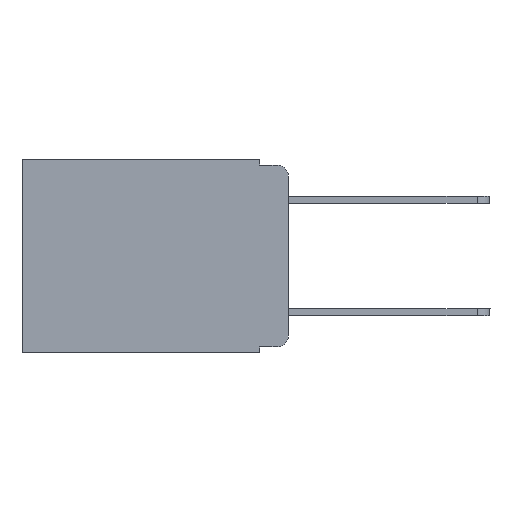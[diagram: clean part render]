
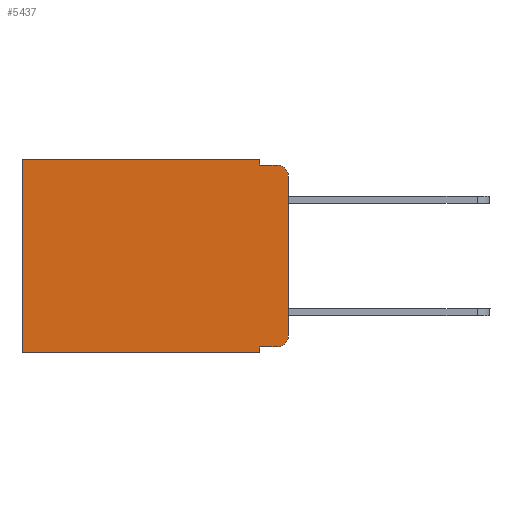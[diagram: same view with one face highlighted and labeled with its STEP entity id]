
A CAD part, left-side view. The second image highlights one B-rep face of the part: STEP entity #5437.
In plain terms, the highlighted planar face has unit normal (-1, 0, 0).
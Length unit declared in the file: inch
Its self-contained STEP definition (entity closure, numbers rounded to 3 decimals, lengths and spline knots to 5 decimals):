
#81 = CIRCLE ( 'NONE', #7023, 0.02 ) ;
#609 = CARTESIAN_POINT ( 'NONE',  ( 0.298, 0., 0. ) ) ;
#875 = DIRECTION ( 'NONE',  ( -1., 0., 0. ) ) ;
#1164 = CARTESIAN_POINT ( 'NONE',  ( 0.298, 0., -0.313 ) ) ;
#1168 = EDGE_CURVE ( 'NONE', #8447, #5330, #4575, .T. ) ;
#1193 = ORIENTED_EDGE ( 'NONE', *, *, #2212, .T. ) ;
#1303 = DIRECTION ( 'NONE',  ( 0., 0., -1. ) ) ;
#1334 = DIRECTION ( 'NONE',  ( 0., 0., -1. ) ) ;
#1465 = LINE ( 'NONE', #5973, #4392 ) ;
#1479 = ORIENTED_EDGE ( 'NONE', *, *, #4085, .F. ) ;
#1498 = DIRECTION ( 'NONE',  ( 0., 0., -1. ) ) ;
#1817 = CARTESIAN_POINT ( 'NONE',  ( 0.298, 0.02, -0.313 ) ) ;
#1825 = EDGE_CURVE ( 'NONE', #5788, #2745, #9775, .T. ) ;
#2212 = EDGE_CURVE ( 'NONE', #3361, #5788, #9214, .T. ) ;
#2239 = ORIENTED_EDGE ( 'NONE', *, *, #1168, .F. ) ;
#2582 = CARTESIAN_POINT ( 'NONE',  ( 0.298, 0.051, -0.333 ) ) ;
#2745 = VERTEX_POINT ( 'NONE', #1164 ) ;
#2805 = LINE ( 'NONE', #609, #9180 ) ;
#2934 = CARTESIAN_POINT ( 'NONE',  ( 0.298, 0.02, -0.03 ) ) ;
#2953 = ORIENTED_EDGE ( 'NONE', *, *, #7912, .T. ) ;
#3233 = LINE ( 'NONE', #3940, #7181 ) ;
#3247 = EDGE_CURVE ( 'NONE', #8263, #9102, #1465, .T. ) ;
#3316 = AXIS2_PLACEMENT_3D ( 'NONE', #1817, #875, #8660 ) ;
#3361 = VERTEX_POINT ( 'NONE', #7774 ) ;
#3495 = DIRECTION ( 'NONE',  ( 0., -1., 0. ) ) ;
#3510 = ORIENTED_EDGE ( 'NONE', *, *, #8692, .F. ) ;
#3664 = VECTOR ( 'NONE', #3495, 39.37008 ) ;
#3793 = CARTESIAN_POINT ( 'NONE',  ( 0.298, 0.051, 0. ) ) ;
#3894 = LINE ( 'NONE', #3793, #7032 ) ;
#3940 = CARTESIAN_POINT ( 'NONE',  ( 0.298, 0., 0. ) ) ;
#4006 = PLANE ( 'NONE',  #4125 ) ;
#4085 = EDGE_CURVE ( 'NONE', #3361, #9686, #7409, .T. ) ;
#4125 = AXIS2_PLACEMENT_3D ( 'NONE', #9094, #4839, #10782 ) ;
#4205 = ORIENTED_EDGE ( 'NONE', *, *, #1825, .T. ) ;
#4349 = CARTESIAN_POINT ( 'NONE',  ( 0.298, 0.473, 0. ) ) ;
#4392 = VECTOR ( 'NONE', #6828, 39.37008 ) ;
#4540 = DIRECTION ( 'NONE',  ( 0., 0., -1. ) ) ;
#4575 = LINE ( 'NONE', #6539, #10565 ) ;
#4653 = DIRECTION ( 'NONE',  ( -1., 0., 0. ) ) ;
#4718 = EDGE_LOOP ( 'NONE', ( #10813, #7399, #2239, #9500, #2953, #8343, #3510, #1479, #1193, #4205 ) ) ;
#4820 = EDGE_CURVE ( 'NONE', #7553, #2745, #2805, .T. ) ;
#4839 = DIRECTION ( 'NONE',  ( 1., 0., 0. ) ) ;
#4878 = DIRECTION ( 'NONE',  ( 0., -1., 0. ) ) ;
#5330 = VERTEX_POINT ( 'NONE', #10750 ) ;
#5437 = ADVANCED_FACE ( 'NONE', ( #6468 ), #4006, .F. ) ;
#5440 = CARTESIAN_POINT ( 'NONE',  ( 0.298, 0.051, -0.343 ) ) ;
#5788 = VERTEX_POINT ( 'NONE', #8857 ) ;
#5789 = EDGE_CURVE ( 'NONE', #7553, #5330, #81, .T. ) ;
#5932 = DIRECTION ( 'NONE',  ( 0., 1., 0. ) ) ;
#5973 = CARTESIAN_POINT ( 'NONE',  ( 0.298, 0.473, 0. ) ) ;
#6303 = CARTESIAN_POINT ( 'NONE',  ( 0.298, 0.051, 0. ) ) ;
#6416 = CARTESIAN_POINT ( 'NONE',  ( 0.298, 0.473, -0.343 ) ) ;
#6468 = FACE_OUTER_BOUND ( 'NONE', #4718, .T. ) ;
#6539 = CARTESIAN_POINT ( 'NONE',  ( 0.298, 0.051, -0.01 ) ) ;
#6828 = DIRECTION ( 'NONE',  ( 0., 0., -1. ) ) ;
#7023 = AXIS2_PLACEMENT_3D ( 'NONE', #2934, #4653, #1303 ) ;
#7032 = VECTOR ( 'NONE', #4540, 39.37008 ) ;
#7159 = VECTOR ( 'NONE', #1334, 39.37008 ) ;
#7181 = VECTOR ( 'NONE', #7205, 39.37008 ) ;
#7205 = DIRECTION ( 'NONE',  ( 0., 1., 0. ) ) ;
#7399 = ORIENTED_EDGE ( 'NONE', *, *, #5789, .T. ) ;
#7409 = LINE ( 'NONE', #6303, #7159 ) ;
#7553 = VERTEX_POINT ( 'NONE', #9924 ) ;
#7774 = CARTESIAN_POINT ( 'NONE',  ( 0.298, 0.051, -0.333 ) ) ;
#7912 = EDGE_CURVE ( 'NONE', #10568, #8263, #3233, .T. ) ;
#8120 = VECTOR ( 'NONE', #5932, 39.37008 ) ;
#8263 = VERTEX_POINT ( 'NONE', #4349 ) ;
#8343 = ORIENTED_EDGE ( 'NONE', *, *, #3247, .T. ) ;
#8447 = VERTEX_POINT ( 'NONE', #9722 ) ;
#8660 = DIRECTION ( 'NONE',  ( 0., 0., -1. ) ) ;
#8692 = EDGE_CURVE ( 'NONE', #9686, #9102, #10400, .T. ) ;
#8711 = CARTESIAN_POINT ( 'NONE',  ( 0.298, 0.051, 0. ) ) ;
#8857 = CARTESIAN_POINT ( 'NONE',  ( 0.298, 0.02, -0.333 ) ) ;
#8982 = EDGE_CURVE ( 'NONE', #10568, #8447, #3894, .T. ) ;
#9094 = CARTESIAN_POINT ( 'NONE',  ( 0.298, 0., 0. ) ) ;
#9102 = VERTEX_POINT ( 'NONE', #6416 ) ;
#9180 = VECTOR ( 'NONE', #1498, 39.37008 ) ;
#9214 = LINE ( 'NONE', #2582, #3664 ) ;
#9500 = ORIENTED_EDGE ( 'NONE', *, *, #8982, .F. ) ;
#9686 = VERTEX_POINT ( 'NONE', #5440 ) ;
#9722 = CARTESIAN_POINT ( 'NONE',  ( 0.298, 0.051, -0.01 ) ) ;
#9775 = CIRCLE ( 'NONE', #3316, 0.02 ) ;
#9924 = CARTESIAN_POINT ( 'NONE',  ( 0.298, 0., -0.03 ) ) ;
#10400 = LINE ( 'NONE', #11011, #8120 ) ;
#10565 = VECTOR ( 'NONE', #4878, 39.37008 ) ;
#10568 = VERTEX_POINT ( 'NONE', #8711 ) ;
#10750 = CARTESIAN_POINT ( 'NONE',  ( 0.298, 0.02, -0.01 ) ) ;
#10782 = DIRECTION ( 'NONE',  ( 0., 0., -1. ) ) ;
#10813 = ORIENTED_EDGE ( 'NONE', *, *, #4820, .F. ) ;
#11011 = CARTESIAN_POINT ( 'NONE',  ( 0.298, 0., -0.343 ) ) ;
